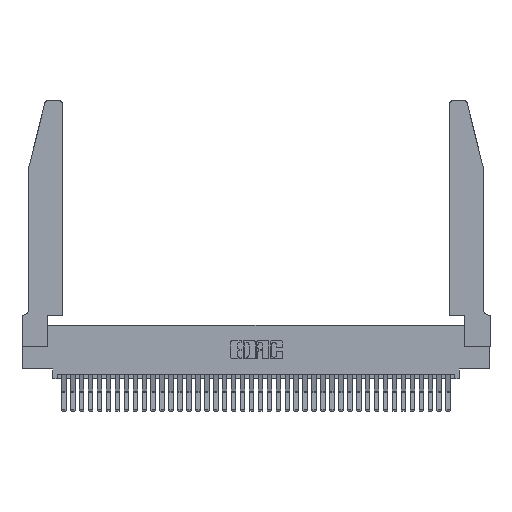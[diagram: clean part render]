
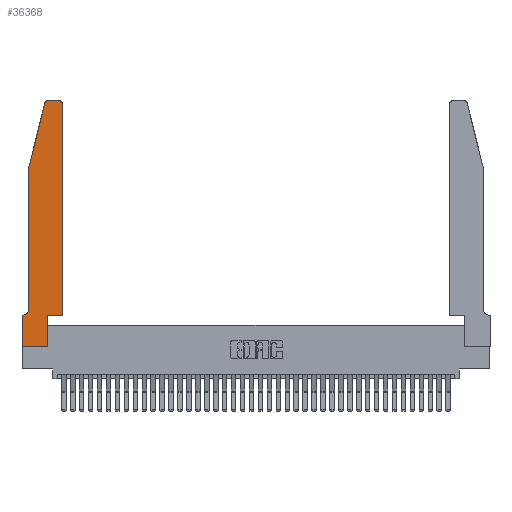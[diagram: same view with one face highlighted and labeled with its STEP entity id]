
A CAD part, top view. The second image highlights one B-rep face of the part: STEP entity #36368.
In plain terms, the highlighted planar face has unit normal (0, 0, 1).
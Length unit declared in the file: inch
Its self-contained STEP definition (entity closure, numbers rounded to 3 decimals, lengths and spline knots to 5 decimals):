
#284 = CARTESIAN_POINT ( 'NONE',  ( 0.0755, 0.42, 0.37 ) ) ;
#960 = CARTESIAN_POINT ( 'NONE',  ( 0.2865, 0.35, 0.37 ) ) ;
#964 = CIRCLE ( 'NONE', #16644, 0.03 ) ;
#965 = CARTESIAN_POINT ( 'NONE',  ( 0.2865, 0., 0.37 ) ) ;
#1029 = ORIENTED_EDGE ( 'NONE', *, *, #29200, .T. ) ;
#1071 = VECTOR ( 'NONE', #21740, 39.37008 ) ;
#1130 = VERTEX_POINT ( 'NONE', #25789 ) ;
#1394 = LINE ( 'NONE', #32108, #24743 ) ;
#1704 = ORIENTED_EDGE ( 'NONE', *, *, #34019, .T. ) ;
#2378 = FACE_OUTER_BOUND ( 'NONE', #16571, .T. ) ;
#2765 = CARTESIAN_POINT ( 'NONE',  ( 0.25487, 2.72718, 0.37 ) ) ;
#2768 = VERTEX_POINT ( 'NONE', #11494 ) ;
#3764 = LINE ( 'NONE', #23141, #9960 ) ;
#3771 = DIRECTION ( 'NONE',  ( 0., 0., -1. ) ) ;
#4204 = LINE ( 'NONE', #20788, #19473 ) ;
#4214 = DIRECTION ( 'NONE',  ( -0.239, -0.971, 0. ) ) ;
#4752 = LINE ( 'NONE', #22454, #20030 ) ;
#4982 = ORIENTED_EDGE ( 'NONE', *, *, #36407, .T. ) ;
#5037 = DIRECTION ( 'NONE',  ( -1., 0., 0. ) ) ;
#5170 = ORIENTED_EDGE ( 'NONE', *, *, #7759, .T. ) ;
#6519 = DIRECTION ( 'NONE',  ( 0., 0., 1. ) ) ;
#7077 = VERTEX_POINT ( 'NONE', #27681 ) ;
#7408 = CARTESIAN_POINT ( 'NONE',  ( 0.4205, 2.75, 0.37 ) ) ;
#7557 = DIRECTION ( 'NONE',  ( 0., 1., 0. ) ) ;
#7759 = EDGE_CURVE ( 'NONE', #2768, #17608, #12184, .T. ) ;
#7848 = PLANE ( 'NONE',  #37248 ) ;
#8225 = DIRECTION ( 'NONE',  ( 0., 0., 1. ) ) ;
#8544 = ORIENTED_EDGE ( 'NONE', *, *, #15911, .T. ) ;
#8584 = DIRECTION ( 'NONE',  ( 1., 0., 0. ) ) ;
#8732 = AXIS2_PLACEMENT_3D ( 'NONE', #24745, #6519, #27767 ) ;
#9146 = VERTEX_POINT ( 'NONE', #960 ) ;
#9231 = CARTESIAN_POINT ( 'NONE',  ( 0.4505, 0.35, 0.37 ) ) ;
#9364 = CARTESIAN_POINT ( 'NONE',  ( 0.2865, 0.35, 0.37 ) ) ;
#9554 = VERTEX_POINT ( 'NONE', #24232 ) ;
#9618 = EDGE_CURVE ( 'NONE', #27354, #9146, #14485, .T. ) ;
#9960 = VECTOR ( 'NONE', #5037, 39.37008 ) ;
#10177 = LINE ( 'NONE', #24774, #1071 ) ;
#10962 = DIRECTION ( 'NONE',  ( 1., 0., 0. ) ) ;
#11484 = ORIENTED_EDGE ( 'NONE', *, *, #23347, .T. ) ;
#11494 = CARTESIAN_POINT ( 'NONE',  ( 0.284, 2.75, 0.37 ) ) ;
#12184 = CIRCLE ( 'NONE', #8732, 0.03 ) ;
#12388 = ORIENTED_EDGE ( 'NONE', *, *, #36237, .T. ) ;
#12838 = VERTEX_POINT ( 'NONE', #284 ) ;
#14485 = LINE ( 'NONE', #9364, #21609 ) ;
#15911 = EDGE_CURVE ( 'NONE', #29512, #2768, #10177, .T. ) ;
#16502 = ORIENTED_EDGE ( 'NONE', *, *, #9618, .T. ) ;
#16571 = EDGE_LOOP ( 'NONE', ( #8544, #5170, #18491, #20766, #12388, #1029, #4982, #17424, #16502, #1704, #11484, #38407 ) ) ;
#16644 = AXIS2_PLACEMENT_3D ( 'NONE', #26417, #8225, #29428 ) ;
#17370 = EDGE_CURVE ( 'NONE', #1130, #29512, #964, .T. ) ;
#17424 = ORIENTED_EDGE ( 'NONE', *, *, #37491, .T. ) ;
#17608 = VERTEX_POINT ( 'NONE', #2765 ) ;
#18491 = ORIENTED_EDGE ( 'NONE', *, *, #21594, .T. ) ;
#18794 = EDGE_CURVE ( 'NONE', #36022, #12838, #4204, .T. ) ;
#19108 = AXIS2_PLACEMENT_3D ( 'NONE', #21998, #3771, #25032 ) ;
#19473 = VECTOR ( 'NONE', #26834, 39.37008 ) ;
#20030 = VECTOR ( 'NONE', #4214, 39.37008 ) ;
#20766 = ORIENTED_EDGE ( 'NONE', *, *, #18794, .T. ) ;
#20788 = CARTESIAN_POINT ( 'NONE',  ( 0.0755, 2., 0.37 ) ) ;
#21594 = EDGE_CURVE ( 'NONE', #17608, #36022, #4752, .T. ) ;
#21609 = VECTOR ( 'NONE', #27384, 39.37008 ) ;
#21740 = DIRECTION ( 'NONE',  ( -1., 0., 0. ) ) ;
#21998 = CARTESIAN_POINT ( 'NONE',  ( 0.0055, 0.42, 0.37 ) ) ;
#22124 = CARTESIAN_POINT ( 'NONE',  ( 0., 0., 0.37 ) ) ;
#22396 = CIRCLE ( 'NONE', #19108, 0.07 ) ;
#22454 = CARTESIAN_POINT ( 'NONE',  ( 0.0755, 2., 0.37 ) ) ;
#23034 = CARTESIAN_POINT ( 'NONE',  ( 0., 0.35, 0.37 ) ) ;
#23141 = CARTESIAN_POINT ( 'NONE',  ( 0.0755, 0.35, 0.37 ) ) ;
#23347 = EDGE_CURVE ( 'NONE', #7077, #1130, #23677, .T. ) ;
#23677 = LINE ( 'NONE', #9231, #30703 ) ;
#24232 = CARTESIAN_POINT ( 'NONE',  ( 0., 0., 0.37 ) ) ;
#24743 = VECTOR ( 'NONE', #38140, 39.37008 ) ;
#24745 = CARTESIAN_POINT ( 'NONE',  ( 0.284, 2.72, 0.37 ) ) ;
#24774 = CARTESIAN_POINT ( 'NONE',  ( 0.2605, 2.75, 0.37 ) ) ;
#25032 = DIRECTION ( 'NONE',  ( -1., 0., 0. ) ) ;
#25158 = DIRECTION ( 'NONE',  ( 1., 0., 0. ) ) ;
#25739 = CARTESIAN_POINT ( 'NONE',  ( 0.0055, 0.35, 0.37 ) ) ;
#25789 = CARTESIAN_POINT ( 'NONE',  ( 0.4505, 2.72, 0.37 ) ) ;
#25800 = CARTESIAN_POINT ( 'NONE',  ( 0., 0.35, 0.37 ) ) ;
#26080 = LINE ( 'NONE', #22124, #34085 ) ;
#26417 = CARTESIAN_POINT ( 'NONE',  ( 0.4205, 2.72, 0.37 ) ) ;
#26834 = DIRECTION ( 'NONE',  ( 0., -1., 0. ) ) ;
#26872 = CARTESIAN_POINT ( 'NONE',  ( 0.0755, 2., 0.37 ) ) ;
#27354 = VERTEX_POINT ( 'NONE', #965 ) ;
#27384 = DIRECTION ( 'NONE',  ( 0., 1., 0. ) ) ;
#27681 = CARTESIAN_POINT ( 'NONE',  ( 0.4505, 0.35, 0.37 ) ) ;
#27767 = DIRECTION ( 'NONE',  ( 1., 0., 0. ) ) ;
#28676 = VECTOR ( 'NONE', #8584, 39.37008 ) ;
#29076 = DIRECTION ( 'NONE',  ( 0., 0., 1. ) ) ;
#29200 = EDGE_CURVE ( 'NONE', #30802, #37659, #3764, .T. ) ;
#29428 = DIRECTION ( 'NONE',  ( 1., 0., 0. ) ) ;
#29512 = VERTEX_POINT ( 'NONE', #7408 ) ;
#29771 = CARTESIAN_POINT ( 'NONE',  ( 0.4505, 0.35, 0.37 ) ) ;
#30562 = LINE ( 'NONE', #29771, #28676 ) ;
#30703 = VECTOR ( 'NONE', #7557, 39.37008 ) ;
#30802 = VERTEX_POINT ( 'NONE', #25739 ) ;
#32108 = CARTESIAN_POINT ( 'NONE',  ( 0., 0., 0.37 ) ) ;
#34019 = EDGE_CURVE ( 'NONE', #9146, #7077, #30562, .T. ) ;
#34085 = VECTOR ( 'NONE', #25158, 39.37008 ) ;
#36022 = VERTEX_POINT ( 'NONE', #26872 ) ;
#36237 = EDGE_CURVE ( 'NONE', #12838, #30802, #22396, .T. ) ;
#36368 = ADVANCED_FACE ( 'NONE', ( #2378 ), #7848, .T. ) ;
#36407 = EDGE_CURVE ( 'NONE', #37659, #9554, #1394, .T. ) ;
#37248 = AXIS2_PLACEMENT_3D ( 'NONE', #23034, #29076, #10962 ) ;
#37491 = EDGE_CURVE ( 'NONE', #9554, #27354, #26080, .T. ) ;
#37659 = VERTEX_POINT ( 'NONE', #25800 ) ;
#38140 = DIRECTION ( 'NONE',  ( 0., -1., 0. ) ) ;
#38407 = ORIENTED_EDGE ( 'NONE', *, *, #17370, .T. ) ;
